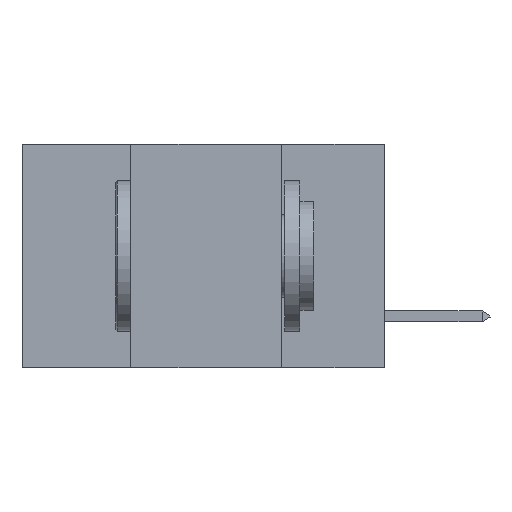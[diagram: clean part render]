
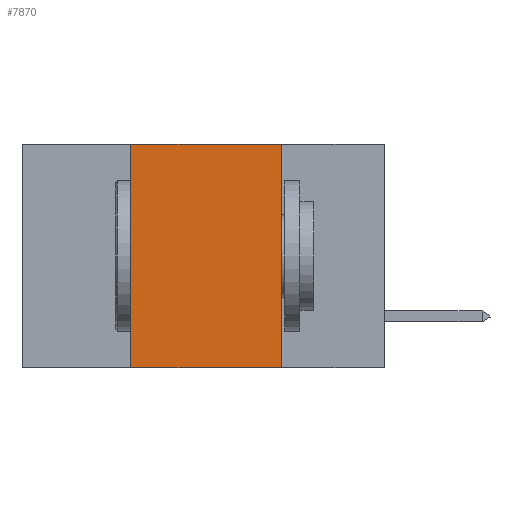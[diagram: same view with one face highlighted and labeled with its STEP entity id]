
A CAD part, left-side view. The second image highlights one B-rep face of the part: STEP entity #7870.
In plain terms, the highlighted planar face has unit normal (-1, 0, 0).
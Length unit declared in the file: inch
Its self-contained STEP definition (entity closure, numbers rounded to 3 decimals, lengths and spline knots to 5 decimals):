
#1131 = FACE_OUTER_BOUND ( 'NONE', #22288, .T. ) ;
#1138 = DIRECTION ( 'NONE',  ( 0., 0., 1. ) ) ;
#1629 = LINE ( 'NONE', #27570, #36886 ) ;
#2301 = DIRECTION ( 'NONE',  ( 0., -1., 0. ) ) ;
#4432 = EDGE_CURVE ( 'NONE', #39263, #40635, #27684, .T. ) ;
#5685 = ORIENTED_EDGE ( 'NONE', *, *, #36922, .F. ) ;
#7870 = ADVANCED_FACE ( 'NONE', ( #1131 ), #36980, .F. ) ;
#8843 = LINE ( 'NONE', #36935, #34182 ) ;
#9104 = ORIENTED_EDGE ( 'NONE', *, *, #4432, .F. ) ;
#9638 = VECTOR ( 'NONE', #23017, 39.37008 ) ;
#11300 = EDGE_CURVE ( 'NONE', #39263, #22061, #1629, .T. ) ;
#11809 = ORIENTED_EDGE ( 'NONE', *, *, #11300, .T. ) ;
#13983 = CARTESIAN_POINT ( 'NONE',  ( 0., 0.17, 0. ) ) ;
#17565 = LINE ( 'NONE', #19798, #9638 ) ;
#19798 = CARTESIAN_POINT ( 'NONE',  ( 0., 0.6, 0. ) ) ;
#22061 = VERTEX_POINT ( 'NONE', #32084 ) ;
#22288 = EDGE_LOOP ( 'NONE', ( #36846, #5685, #9104, #11809 ) ) ;
#23017 = DIRECTION ( 'NONE',  ( 0., -1., 0. ) ) ;
#27181 = CARTESIAN_POINT ( 'NONE',  ( 0., 0.42, 0. ) ) ;
#27344 = VERTEX_POINT ( 'NONE', #13983 ) ;
#27570 = CARTESIAN_POINT ( 'NONE',  ( 0., 0.6, -0.37 ) ) ;
#27623 = DIRECTION ( 'NONE',  ( 0., 0., -1. ) ) ;
#27684 = LINE ( 'NONE', #32687, #30618 ) ;
#30049 = CARTESIAN_POINT ( 'NONE',  ( 0., 0.6, 0. ) ) ;
#30234 = AXIS2_PLACEMENT_3D ( 'NONE', #30049, #34614, #27623 ) ;
#30618 = VECTOR ( 'NONE', #1138, 39.37008 ) ;
#32084 = CARTESIAN_POINT ( 'NONE',  ( 0., 0.17, -0.37 ) ) ;
#32375 = CARTESIAN_POINT ( 'NONE',  ( 0., 0.42, -0.37 ) ) ;
#32687 = CARTESIAN_POINT ( 'NONE',  ( 0., 0.42, 0. ) ) ;
#34182 = VECTOR ( 'NONE', #36793, 39.37008 ) ;
#34614 = DIRECTION ( 'NONE',  ( 1., 0., 0. ) ) ;
#36793 = DIRECTION ( 'NONE',  ( 0., 0., -1. ) ) ;
#36846 = ORIENTED_EDGE ( 'NONE', *, *, #40186, .F. ) ;
#36886 = VECTOR ( 'NONE', #2301, 39.37008 ) ;
#36922 = EDGE_CURVE ( 'NONE', #40635, #27344, #17565, .T. ) ;
#36935 = CARTESIAN_POINT ( 'NONE',  ( 0., 0.17, 0. ) ) ;
#36980 = PLANE ( 'NONE',  #30234 ) ;
#39263 = VERTEX_POINT ( 'NONE', #32375 ) ;
#40186 = EDGE_CURVE ( 'NONE', #27344, #22061, #8843, .T. ) ;
#40635 = VERTEX_POINT ( 'NONE', #27181 ) ;
